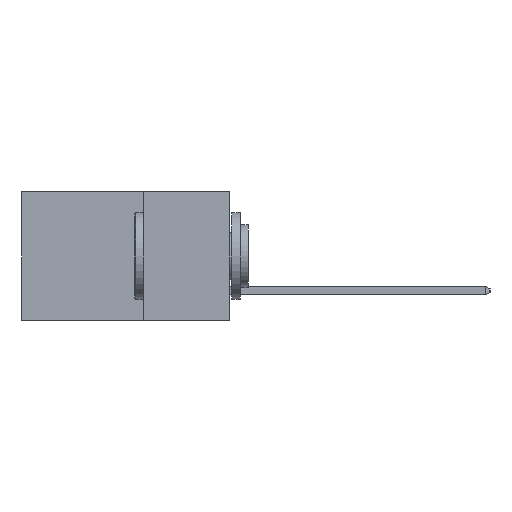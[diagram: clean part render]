
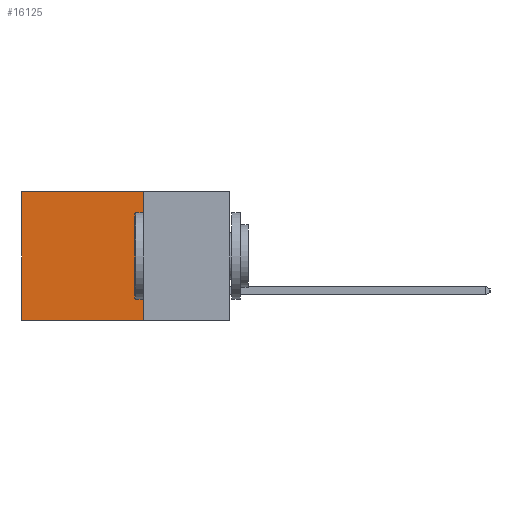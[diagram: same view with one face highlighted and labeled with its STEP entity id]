
A CAD part, left-side view. The second image highlights one B-rep face of the part: STEP entity #16125.
In plain terms, the highlighted planar face has unit normal (-1, 0, 0).
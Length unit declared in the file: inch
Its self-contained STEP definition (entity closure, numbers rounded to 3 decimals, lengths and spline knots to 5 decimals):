
#77 = EDGE_LOOP ( 'NONE', ( #6544, #21617, #7741, #4117 ) ) ;
#3500 = EDGE_CURVE ( 'NONE', #12184, #12546, #13826, .T. ) ;
#3603 = DIRECTION ( 'NONE',  ( 0., 1., 0. ) ) ;
#3774 = EDGE_CURVE ( 'NONE', #13852, #15630, #12368, .T. ) ;
#3828 = CARTESIAN_POINT ( 'NONE',  ( 0.2615, 0.25, -0.37 ) ) ;
#4117 = ORIENTED_EDGE ( 'NONE', *, *, #19277, .T. ) ;
#6544 = ORIENTED_EDGE ( 'NONE', *, *, #3500, .T. ) ;
#7107 = CARTESIAN_POINT ( 'NONE',  ( 0.2615, 0.6, -0.37 ) ) ;
#7257 = DIRECTION ( 'NONE',  ( 0., 0., -1. ) ) ;
#7741 = ORIENTED_EDGE ( 'NONE', *, *, #3774, .F. ) ;
#8804 = CARTESIAN_POINT ( 'NONE',  ( 0.2615, 0.6, 0. ) ) ;
#9887 = LINE ( 'NONE', #3828, #14830 ) ;
#9894 = CARTESIAN_POINT ( 'NONE',  ( 0.2615, 0.6, -0.37 ) ) ;
#11779 = CARTESIAN_POINT ( 'NONE',  ( 0.2615, 0.25, -0.37 ) ) ;
#11783 = VECTOR ( 'NONE', #16319, 39.37008 ) ;
#12184 = VERTEX_POINT ( 'NONE', #8804 ) ;
#12368 = LINE ( 'NONE', #16903, #11783 ) ;
#12546 = VERTEX_POINT ( 'NONE', #9894 ) ;
#13767 = CARTESIAN_POINT ( 'NONE',  ( 0.2615, 0.25, 0. ) ) ;
#13826 = LINE ( 'NONE', #7107, #22802 ) ;
#13852 = VERTEX_POINT ( 'NONE', #13855 ) ;
#13855 = CARTESIAN_POINT ( 'NONE',  ( 0.2615, 0.25, 0. ) ) ;
#14830 = VECTOR ( 'NONE', #3603, 39.37008 ) ;
#15630 = VERTEX_POINT ( 'NONE', #11779 ) ;
#16125 = ADVANCED_FACE ( 'NONE', ( #22945 ), #21659, .F. ) ;
#16319 = DIRECTION ( 'NONE',  ( 0., 0., -1. ) ) ;
#16903 = CARTESIAN_POINT ( 'NONE',  ( 0.2615, 0.25, -0.37 ) ) ;
#17521 = EDGE_CURVE ( 'NONE', #15630, #12546, #9887, .T. ) ;
#18413 = VECTOR ( 'NONE', #22711, 39.37008 ) ;
#19277 = EDGE_CURVE ( 'NONE', #13852, #12184, #22539, .T. ) ;
#20146 = AXIS2_PLACEMENT_3D ( 'NONE', #21706, #21633, #21609 ) ;
#21609 = DIRECTION ( 'NONE',  ( 0., 0., -1. ) ) ;
#21617 = ORIENTED_EDGE ( 'NONE', *, *, #17521, .F. ) ;
#21633 = DIRECTION ( 'NONE',  ( 1., 0., 0. ) ) ;
#21659 = PLANE ( 'NONE',  #20146 ) ;
#21706 = CARTESIAN_POINT ( 'NONE',  ( 0.2615, 0.25, -0.37 ) ) ;
#22539 = LINE ( 'NONE', #13767, #18413 ) ;
#22711 = DIRECTION ( 'NONE',  ( 0., 1., 0. ) ) ;
#22802 = VECTOR ( 'NONE', #7257, 39.37008 ) ;
#22945 = FACE_OUTER_BOUND ( 'NONE', #77, .T. ) ;
